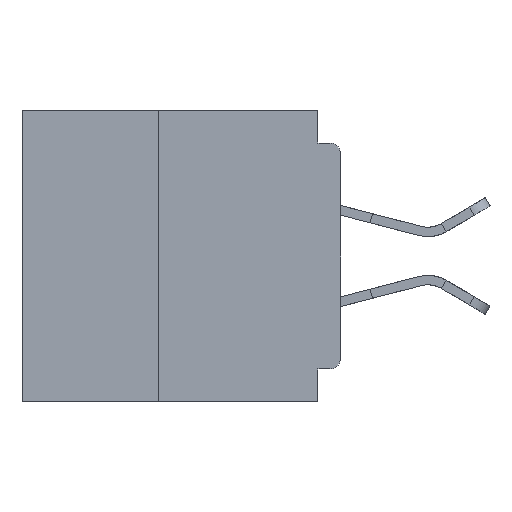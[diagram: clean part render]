
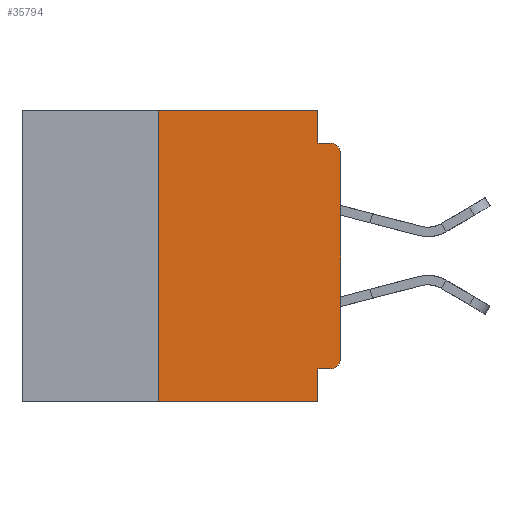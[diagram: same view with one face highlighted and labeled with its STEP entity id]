
A CAD part, left-side view. The second image highlights one B-rep face of the part: STEP entity #35794.
In plain terms, the highlighted planar face has unit normal (-1, 0, 0).
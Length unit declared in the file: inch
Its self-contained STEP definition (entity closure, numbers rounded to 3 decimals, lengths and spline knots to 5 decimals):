
#210 = VERTEX_POINT ( 'NONE', #22181 ) ;
#404 = CIRCLE ( 'NONE', #5403, 0.015 ) ;
#1880 = LINE ( 'NONE', #28409, #25021 ) ;
#2101 = CARTESIAN_POINT ( 'NONE',  ( 0., 0.015, -0.045 ) ) ;
#2620 = ORIENTED_EDGE ( 'NONE', *, *, #15760, .T. ) ;
#2948 = CARTESIAN_POINT ( 'NONE',  ( 0., 0., -0.06 ) ) ;
#3086 = ORIENTED_EDGE ( 'NONE', *, *, #26106, .F. ) ;
#3125 = EDGE_CURVE ( 'NONE', #15862, #18859, #1880, .T. ) ;
#3321 = VECTOR ( 'NONE', #3337, 39.37008 ) ;
#3337 = DIRECTION ( 'NONE',  ( 0., 0., -1. ) ) ;
#4094 = EDGE_CURVE ( 'NONE', #210, #15862, #28470, .T. ) ;
#4204 = LINE ( 'NONE', #18321, #11447 ) ;
#4362 = DIRECTION ( 'NONE',  ( 0., -1., 0. ) ) ;
#4368 = DIRECTION ( 'NONE',  ( 0., 1., 0. ) ) ;
#5158 = DIRECTION ( 'NONE',  ( 0., 0., -1. ) ) ;
#5204 = CARTESIAN_POINT ( 'NONE',  ( 0., 0.031, -0.355 ) ) ;
#5403 = AXIS2_PLACEMENT_3D ( 'NONE', #13462, #33974, #16448 ) ;
#7957 = LINE ( 'NONE', #28445, #22924 ) ;
#8506 = EDGE_LOOP ( 'NONE', ( #34888, #2620, #32312, #32485, #37438, #30757, #27201, #34114, #3086, #30155 ) ) ;
#10242 = DIRECTION ( 'NONE',  ( -1., 0., 0. ) ) ;
#10582 = CARTESIAN_POINT ( 'NONE',  ( 0., 0., -0.355 ) ) ;
#11447 = VECTOR ( 'NONE', #21265, 39.37008 ) ;
#12176 = CARTESIAN_POINT ( 'NONE',  ( 0., 0.25, -0.4 ) ) ;
#12448 = FACE_OUTER_BOUND ( 'NONE', #8506, .T. ) ;
#12785 = VECTOR ( 'NONE', #15356, 39.37008 ) ;
#13462 = CARTESIAN_POINT ( 'NONE',  ( 0., 0.015, -0.34 ) ) ;
#14297 = CIRCLE ( 'NONE', #22999, 0.015 ) ;
#15356 = DIRECTION ( 'NONE',  ( 0., -1., 0. ) ) ;
#15760 = EDGE_CURVE ( 'NONE', #35994, #32571, #14297, .T. ) ;
#15862 = VERTEX_POINT ( 'NONE', #19632 ) ;
#15996 = LINE ( 'NONE', #17011, #38254 ) ;
#16448 = DIRECTION ( 'NONE',  ( 0., 0., -1. ) ) ;
#16628 = CARTESIAN_POINT ( 'NONE',  ( 0., 0.437, -0.4 ) ) ;
#17011 = CARTESIAN_POINT ( 'NONE',  ( 0., 0.25, -0.4 ) ) ;
#17236 = PLANE ( 'NONE',  #38004 ) ;
#17422 = VERTEX_POINT ( 'NONE', #24055 ) ;
#18321 = CARTESIAN_POINT ( 'NONE',  ( 0., 0., 0. ) ) ;
#18859 = VERTEX_POINT ( 'NONE', #34300 ) ;
#19632 = CARTESIAN_POINT ( 'NONE',  ( 0., 0.031, 0. ) ) ;
#20131 = LINE ( 'NONE', #16628, #34730 ) ;
#20196 = CARTESIAN_POINT ( 'NONE',  ( 0., 0.437, 0. ) ) ;
#21265 = DIRECTION ( 'NONE',  ( 0., 0., 1. ) ) ;
#22181 = CARTESIAN_POINT ( 'NONE',  ( 0., 0.25, 0. ) ) ;
#22924 = VECTOR ( 'NONE', #31357, 39.37008 ) ;
#22999 = AXIS2_PLACEMENT_3D ( 'NONE', #28004, #10242, #30921 ) ;
#23160 = DIRECTION ( 'NONE',  ( 1., 0., 0. ) ) ;
#23253 = EDGE_CURVE ( 'NONE', #26430, #29293, #20131, .T. ) ;
#24055 = CARTESIAN_POINT ( 'NONE',  ( 0., 0., -0.34 ) ) ;
#24555 = CARTESIAN_POINT ( 'NONE',  ( 0., 0.031, -0.4 ) ) ;
#24878 = EDGE_CURVE ( 'NONE', #33124, #17422, #404, .T. ) ;
#25021 = VECTOR ( 'NONE', #28372, 39.37008 ) ;
#25261 = EDGE_CURVE ( 'NONE', #27759, #29293, #34079, .T. ) ;
#25652 = CARTESIAN_POINT ( 'NONE',  ( 0., 0.015, -0.355 ) ) ;
#26106 = EDGE_CURVE ( 'NONE', #33124, #27759, #34011, .T. ) ;
#26341 = VECTOR ( 'NONE', #4368, 39.37008 ) ;
#26430 = VERTEX_POINT ( 'NONE', #12176 ) ;
#27122 = CARTESIAN_POINT ( 'NONE',  ( 0., 0.437, 0. ) ) ;
#27201 = ORIENTED_EDGE ( 'NONE', *, *, #23253, .T. ) ;
#27759 = VERTEX_POINT ( 'NONE', #5204 ) ;
#28004 = CARTESIAN_POINT ( 'NONE',  ( 0., 0.015, -0.06 ) ) ;
#28372 = DIRECTION ( 'NONE',  ( 0., 0., -1. ) ) ;
#28409 = CARTESIAN_POINT ( 'NONE',  ( 0., 0.031, 0. ) ) ;
#28445 = CARTESIAN_POINT ( 'NONE',  ( 0., 0., -0.045 ) ) ;
#28470 = LINE ( 'NONE', #27122, #12785 ) ;
#28830 = DIRECTION ( 'NONE',  ( 0., 0., 1. ) ) ;
#29293 = VERTEX_POINT ( 'NONE', #33267 ) ;
#30155 = ORIENTED_EDGE ( 'NONE', *, *, #24878, .T. ) ;
#30757 = ORIENTED_EDGE ( 'NONE', *, *, #33172, .F. ) ;
#30921 = DIRECTION ( 'NONE',  ( 0., 0., -1. ) ) ;
#31357 = DIRECTION ( 'NONE',  ( 0., -1., 0. ) ) ;
#31529 = EDGE_CURVE ( 'NONE', #17422, #35994, #4204, .T. ) ;
#32312 = ORIENTED_EDGE ( 'NONE', *, *, #38320, .F. ) ;
#32485 = ORIENTED_EDGE ( 'NONE', *, *, #3125, .F. ) ;
#32571 = VERTEX_POINT ( 'NONE', #2101 ) ;
#33124 = VERTEX_POINT ( 'NONE', #25652 ) ;
#33172 = EDGE_CURVE ( 'NONE', #26430, #210, #15996, .T. ) ;
#33267 = CARTESIAN_POINT ( 'NONE',  ( 0., 0.031, -0.4 ) ) ;
#33974 = DIRECTION ( 'NONE',  ( -1., 0., 0. ) ) ;
#34011 = LINE ( 'NONE', #10582, #26341 ) ;
#34079 = LINE ( 'NONE', #24555, #3321 ) ;
#34114 = ORIENTED_EDGE ( 'NONE', *, *, #25261, .F. ) ;
#34300 = CARTESIAN_POINT ( 'NONE',  ( 0., 0.031, -0.045 ) ) ;
#34730 = VECTOR ( 'NONE', #4362, 39.37008 ) ;
#34888 = ORIENTED_EDGE ( 'NONE', *, *, #31529, .T. ) ;
#35794 = ADVANCED_FACE ( 'NONE', ( #12448 ), #17236, .F. ) ;
#35994 = VERTEX_POINT ( 'NONE', #2948 ) ;
#37438 = ORIENTED_EDGE ( 'NONE', *, *, #4094, .F. ) ;
#38004 = AXIS2_PLACEMENT_3D ( 'NONE', #20196, #23160, #5158 ) ;
#38254 = VECTOR ( 'NONE', #28830, 39.37008 ) ;
#38320 = EDGE_CURVE ( 'NONE', #18859, #32571, #7957, .T. ) ;
